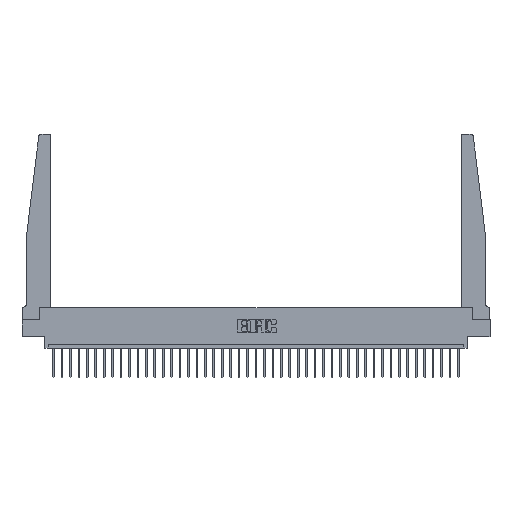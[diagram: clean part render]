
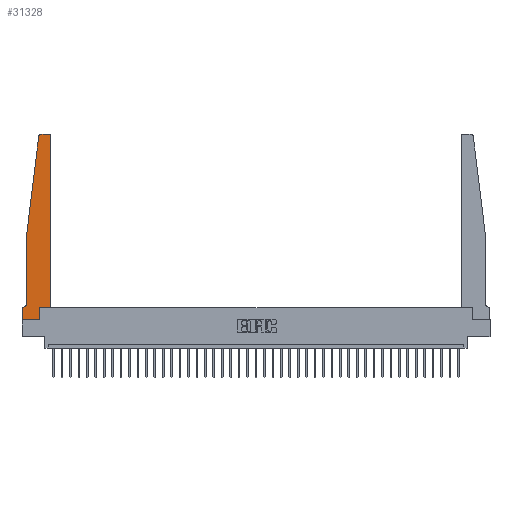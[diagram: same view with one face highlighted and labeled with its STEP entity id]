
A CAD part, top view. The second image highlights one B-rep face of the part: STEP entity #31328.
In plain terms, the highlighted planar face has unit normal (0, 0, 1).
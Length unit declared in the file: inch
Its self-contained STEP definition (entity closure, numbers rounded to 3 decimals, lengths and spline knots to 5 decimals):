
#242 = CARTESIAN_POINT ( 'NONE',  ( 0.065, 1.25, 0.37 ) ) ;
#553 = CIRCLE ( 'NONE', #11981, 0.03 ) ;
#755 = CARTESIAN_POINT ( 'NONE',  ( 0.015, 0.1875, 0.37 ) ) ;
#900 = CARTESIAN_POINT ( 'NONE',  ( 0.395, 2.75, 0.37 ) ) ;
#1222 = ORIENTED_EDGE ( 'NONE', *, *, #28349, .T. ) ;
#1296 = LINE ( 'NONE', #25246, #28734 ) ;
#1605 = DIRECTION ( 'NONE',  ( 0., 0., 1. ) ) ;
#1689 = FACE_OUTER_BOUND ( 'NONE', #4060, .T. ) ;
#2022 = CARTESIAN_POINT ( 'NONE',  ( 0.25, 2.75, 0.37 ) ) ;
#2958 = DIRECTION ( 'NONE',  ( 1., 0., 0. ) ) ;
#2968 = EDGE_CURVE ( 'NONE', #4989, #22475, #19543, .T. ) ;
#3298 = CARTESIAN_POINT ( 'NONE',  ( 0.27653, 2.75, 0.37 ) ) ;
#3842 = ORIENTED_EDGE ( 'NONE', *, *, #27185, .T. ) ;
#3964 = CARTESIAN_POINT ( 'NONE',  ( 0., 0.1875, 0.37 ) ) ;
#4060 = EDGE_LOOP ( 'NONE', ( #13816, #1222, #10192, #30993, #27028, #10661, #10004, #3842, #30050, #14899, #31404, #33302 ) ) ;
#4419 = LINE ( 'NONE', #8108, #22305 ) ;
#4638 = VECTOR ( 'NONE', #6461, 39.37008 ) ;
#4989 = VERTEX_POINT ( 'NONE', #25677 ) ;
#5390 = CARTESIAN_POINT ( 'NONE',  ( 0., 0., 0.37 ) ) ;
#6315 = DIRECTION ( 'NONE',  ( 1., 0., 0. ) ) ;
#6461 = DIRECTION ( 'NONE',  ( 0., -1., 0. ) ) ;
#6604 = CARTESIAN_POINT ( 'NONE',  ( 0.395, 2.72, 0.37 ) ) ;
#6630 = VERTEX_POINT ( 'NONE', #900 ) ;
#7041 = EDGE_CURVE ( 'NONE', #13883, #32836, #26270, .T. ) ;
#7655 = CIRCLE ( 'NONE', #8967, 0.05 ) ;
#8010 = LINE ( 'NONE', #22251, #4638 ) ;
#8108 = CARTESIAN_POINT ( 'NONE',  ( 0., 0., 0.37 ) ) ;
#8514 = EDGE_CURVE ( 'NONE', #18190, #16413, #8010, .T. ) ;
#8837 = VERTEX_POINT ( 'NONE', #27943 ) ;
#8967 = AXIS2_PLACEMENT_3D ( 'NONE', #11533, #21807, #13944 ) ;
#9433 = LINE ( 'NONE', #17456, #27254 ) ;
#9631 = EDGE_CURVE ( 'NONE', #17153, #6630, #11363, .T. ) ;
#9920 = EDGE_CURVE ( 'NONE', #22475, #17153, #1296, .T. ) ;
#10004 = ORIENTED_EDGE ( 'NONE', *, *, #8514, .T. ) ;
#10192 = ORIENTED_EDGE ( 'NONE', *, *, #7041, .T. ) ;
#10661 = ORIENTED_EDGE ( 'NONE', *, *, #13541, .T. ) ;
#11195 = VECTOR ( 'NONE', #25476, 39.37008 ) ;
#11363 = CIRCLE ( 'NONE', #25156, 0.03 ) ;
#11533 = CARTESIAN_POINT ( 'NONE',  ( 0.015, 0.2375, 0.37 ) ) ;
#11583 = CARTESIAN_POINT ( 'NONE',  ( 0., 0.1875, 0.37 ) ) ;
#11614 = DIRECTION ( 'NONE',  ( 0., -1., 0. ) ) ;
#11760 = EDGE_CURVE ( 'NONE', #6630, #16643, #12047, .T. ) ;
#11981 = AXIS2_PLACEMENT_3D ( 'NONE', #14882, #1605, #22895 ) ;
#12047 = LINE ( 'NONE', #2022, #11195 ) ;
#12410 = CARTESIAN_POINT ( 'NONE',  ( 0.065, 1.25, 0.37 ) ) ;
#13259 = VERTEX_POINT ( 'NONE', #20120 ) ;
#13541 = EDGE_CURVE ( 'NONE', #28773, #18190, #18923, .T. ) ;
#13816 = ORIENTED_EDGE ( 'NONE', *, *, #11760, .T. ) ;
#13883 = VERTEX_POINT ( 'NONE', #31611 ) ;
#13944 = DIRECTION ( 'NONE',  ( -1., 0., 0. ) ) ;
#14882 = CARTESIAN_POINT ( 'NONE',  ( 0.27653, 2.72, 0.37 ) ) ;
#14899 = ORIENTED_EDGE ( 'NONE', *, *, #2968, .T. ) ;
#15118 = LINE ( 'NONE', #242, #17599 ) ;
#15536 = AXIS2_PLACEMENT_3D ( 'NONE', #11583, #24742, #6315 ) ;
#16209 = DIRECTION ( 'NONE',  ( 1., 0., 0. ) ) ;
#16413 = VERTEX_POINT ( 'NONE', #5390 ) ;
#16569 = DIRECTION ( 'NONE',  ( 1., 0., 0. ) ) ;
#16643 = VERTEX_POINT ( 'NONE', #3298 ) ;
#17153 = VERTEX_POINT ( 'NONE', #32381 ) ;
#17456 = CARTESIAN_POINT ( 'NONE',  ( 0.2605, 0.18, 0.37 ) ) ;
#17599 = VECTOR ( 'NONE', #11614, 39.37008 ) ;
#18190 = VERTEX_POINT ( 'NONE', #3964 ) ;
#18923 = LINE ( 'NONE', #31067, #31715 ) ;
#19543 = LINE ( 'NONE', #23886, #19965 ) ;
#19890 = PLANE ( 'NONE',  #15536 ) ;
#19965 = VECTOR ( 'NONE', #2958, 39.37008 ) ;
#20120 = CARTESIAN_POINT ( 'NONE',  ( 0.065, 0.2375, 0.37 ) ) ;
#20480 = EDGE_CURVE ( 'NONE', #32836, #13259, #15118, .T. ) ;
#20709 = DIRECTION ( 'NONE',  ( -0.122, -0.992, 0. ) ) ;
#21792 = DIRECTION ( 'NONE',  ( -1., 0., 0. ) ) ;
#21807 = DIRECTION ( 'NONE',  ( 0., 0., -1. ) ) ;
#22230 = EDGE_CURVE ( 'NONE', #13259, #28773, #7655, .T. ) ;
#22251 = CARTESIAN_POINT ( 'NONE',  ( 0., 0., 0.37 ) ) ;
#22305 = VECTOR ( 'NONE', #16209, 39.37008 ) ;
#22475 = VERTEX_POINT ( 'NONE', #22730 ) ;
#22730 = CARTESIAN_POINT ( 'NONE',  ( 0.425, 0.18, 0.37 ) ) ;
#22895 = DIRECTION ( 'NONE',  ( 1., 0., 0. ) ) ;
#23155 = DIRECTION ( 'NONE',  ( 0., 1., 0. ) ) ;
#23886 = CARTESIAN_POINT ( 'NONE',  ( 0.425, 0.18, 0.37 ) ) ;
#24742 = DIRECTION ( 'NONE',  ( 0., 0., 1. ) ) ;
#25156 = AXIS2_PLACEMENT_3D ( 'NONE', #6604, #27927, #16569 ) ;
#25246 = CARTESIAN_POINT ( 'NONE',  ( 0.425, 0.18, 0.37 ) ) ;
#25476 = DIRECTION ( 'NONE',  ( -1., 0., 0. ) ) ;
#25677 = CARTESIAN_POINT ( 'NONE',  ( 0.2605, 0.18, 0.37 ) ) ;
#26270 = LINE ( 'NONE', #33320, #31636 ) ;
#27028 = ORIENTED_EDGE ( 'NONE', *, *, #22230, .T. ) ;
#27185 = EDGE_CURVE ( 'NONE', #16413, #8837, #4419, .T. ) ;
#27254 = VECTOR ( 'NONE', #23155, 39.37008 ) ;
#27642 = EDGE_CURVE ( 'NONE', #8837, #4989, #9433, .T. ) ;
#27927 = DIRECTION ( 'NONE',  ( 0., 0., 1. ) ) ;
#27943 = CARTESIAN_POINT ( 'NONE',  ( 0.2605, 0., 0.37 ) ) ;
#28349 = EDGE_CURVE ( 'NONE', #16643, #13883, #553, .T. ) ;
#28734 = VECTOR ( 'NONE', #33459, 39.37008 ) ;
#28773 = VERTEX_POINT ( 'NONE', #755 ) ;
#30050 = ORIENTED_EDGE ( 'NONE', *, *, #27642, .T. ) ;
#30993 = ORIENTED_EDGE ( 'NONE', *, *, #20480, .T. ) ;
#31067 = CARTESIAN_POINT ( 'NONE',  ( 0.065, 0.1875, 0.37 ) ) ;
#31328 = ADVANCED_FACE ( 'NONE', ( #1689 ), #19890, .T. ) ;
#31404 = ORIENTED_EDGE ( 'NONE', *, *, #9920, .T. ) ;
#31611 = CARTESIAN_POINT ( 'NONE',  ( 0.24675, 2.72367, 0.37 ) ) ;
#31636 = VECTOR ( 'NONE', #20709, 39.37008 ) ;
#31715 = VECTOR ( 'NONE', #21792, 39.37008 ) ;
#32381 = CARTESIAN_POINT ( 'NONE',  ( 0.425, 2.72, 0.37 ) ) ;
#32836 = VERTEX_POINT ( 'NONE', #12410 ) ;
#33302 = ORIENTED_EDGE ( 'NONE', *, *, #9631, .T. ) ;
#33320 = CARTESIAN_POINT ( 'NONE',  ( 0.065, 1.25, 0.37 ) ) ;
#33459 = DIRECTION ( 'NONE',  ( 0., 1., 0. ) ) ;
